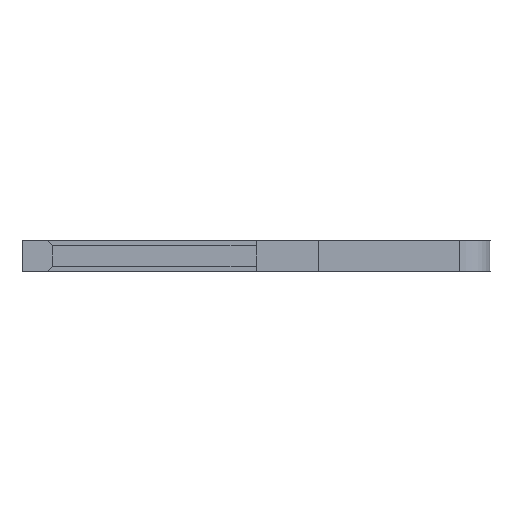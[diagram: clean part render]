
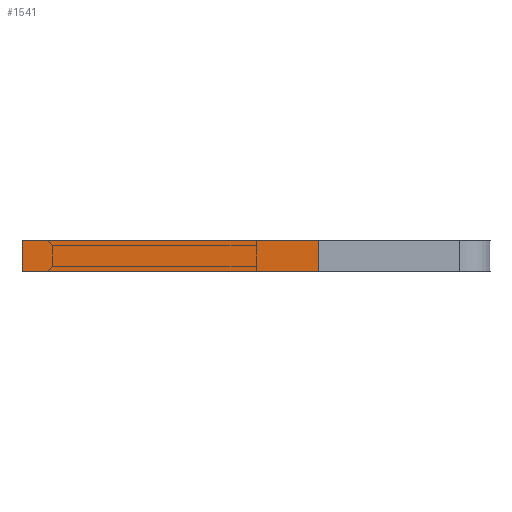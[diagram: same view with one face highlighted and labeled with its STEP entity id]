
A CAD part, left-side view. The second image highlights one B-rep face of the part: STEP entity #1541.
In plain terms, the highlighted face is planar.
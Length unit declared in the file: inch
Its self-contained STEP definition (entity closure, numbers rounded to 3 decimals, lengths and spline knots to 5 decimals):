
#75 = EDGE_CURVE ( 'NONE', #1594, #1250, #1058, .T. ) ;
#130 = ORIENTED_EDGE ( 'NONE', *, *, #2078, .F. ) ;
#148 = CARTESIAN_POINT ( 'NONE',  ( -0.01, 0.15, -0.04 ) ) ;
#182 = VECTOR ( 'NONE', #1666, 39.37008 ) ;
#215 = VECTOR ( 'NONE', #2216, 39.37008 ) ;
#359 = CARTESIAN_POINT ( 'NONE',  ( 0.01, -0.04, -0.04 ) ) ;
#419 = CARTESIAN_POINT ( 'NONE',  ( 0.01, -0.04, -0.04 ) ) ;
#474 = FACE_OUTER_BOUND ( 'NONE', #1025, .T. ) ;
#713 = LINE ( 'NONE', #800, #722 ) ;
#722 = VECTOR ( 'NONE', #2385, 39.37008 ) ;
#800 = CARTESIAN_POINT ( 'NONE',  ( 0.01, 0.15, -0.04 ) ) ;
#881 = VERTEX_POINT ( 'NONE', #1322 ) ;
#933 = DIRECTION ( 'NONE',  ( 1., 0., 0. ) ) ;
#1025 = EDGE_LOOP ( 'NONE', ( #2469, #1132, #130, #2049 ) ) ;
#1052 = EDGE_CURVE ( 'NONE', #881, #1353, #2369, .T. ) ;
#1058 = LINE ( 'NONE', #419, #215 ) ;
#1132 = ORIENTED_EDGE ( 'NONE', *, *, #1052, .F. ) ;
#1155 = CARTESIAN_POINT ( 'NONE',  ( 0.01, 0.15, -0.04 ) ) ;
#1161 = EDGE_CURVE ( 'NONE', #1250, #1353, #2461, .T. ) ;
#1250 = VERTEX_POINT ( 'NONE', #1702 ) ;
#1322 = CARTESIAN_POINT ( 'NONE',  ( 0.01, 0.15, -0.04 ) ) ;
#1353 = VERTEX_POINT ( 'NONE', #1366 ) ;
#1366 = CARTESIAN_POINT ( 'NONE',  ( -0.01, 0.15, -0.04 ) ) ;
#1541 = ADVANCED_FACE ( 'NONE', ( #474 ), #2143, .F. ) ;
#1594 = VERTEX_POINT ( 'NONE', #359 ) ;
#1666 = DIRECTION ( 'NONE',  ( -1., 0., 0. ) ) ;
#1702 = CARTESIAN_POINT ( 'NONE',  ( -0.01, -0.04, -0.04 ) ) ;
#1891 = CARTESIAN_POINT ( 'NONE',  ( 0.01, 0.15, -0.04 ) ) ;
#1937 = AXIS2_PLACEMENT_3D ( 'NONE', #1155, #2339, #933 ) ;
#2049 = ORIENTED_EDGE ( 'NONE', *, *, #75, .T. ) ;
#2078 = EDGE_CURVE ( 'NONE', #1594, #881, #713, .T. ) ;
#2126 = DIRECTION ( 'NONE',  ( 0., 1., 0. ) ) ;
#2143 = PLANE ( 'NONE',  #1937 ) ;
#2216 = DIRECTION ( 'NONE',  ( -1., 0., 0. ) ) ;
#2245 = VECTOR ( 'NONE', #2126, 39.37008 ) ;
#2339 = DIRECTION ( 'NONE',  ( 0., 0., 1. ) ) ;
#2369 = LINE ( 'NONE', #1891, #182 ) ;
#2385 = DIRECTION ( 'NONE',  ( 0., 1., 0. ) ) ;
#2461 = LINE ( 'NONE', #148, #2245 ) ;
#2469 = ORIENTED_EDGE ( 'NONE', *, *, #1161, .T. ) ;
